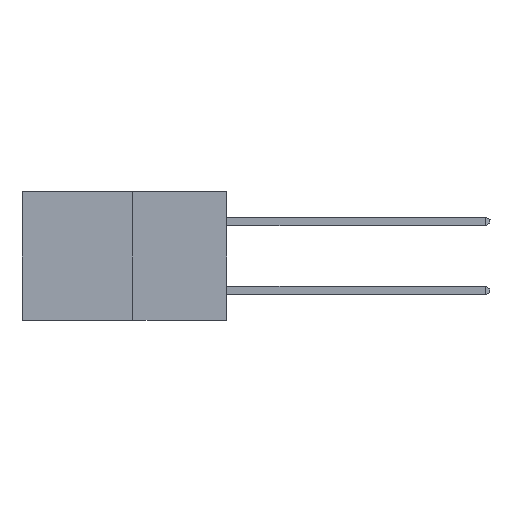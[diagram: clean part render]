
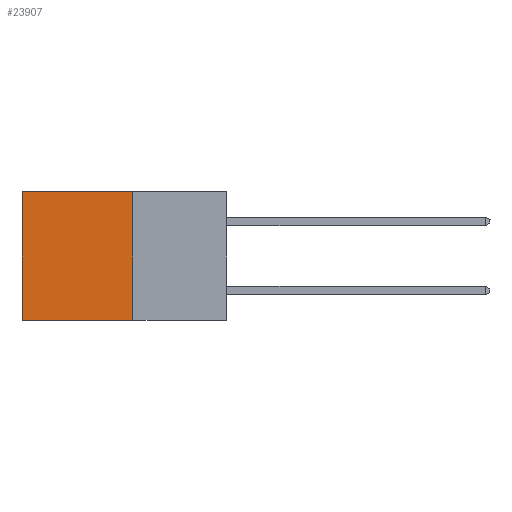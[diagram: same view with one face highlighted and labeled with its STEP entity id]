
A CAD part, left-side view. The second image highlights one B-rep face of the part: STEP entity #23907.
In plain terms, the highlighted planar face has unit normal (-1, 0, 0).
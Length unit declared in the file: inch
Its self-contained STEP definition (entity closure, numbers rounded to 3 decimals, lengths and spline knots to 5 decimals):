
#242 = DIRECTION ( 'NONE',  ( 0., 1., 0. ) ) ;
#1425 = EDGE_CURVE ( 'NONE', #26429, #18864, #28912, .T. ) ;
#3086 = VECTOR ( 'NONE', #17994, 39.37008 ) ;
#3312 = DIRECTION ( 'NONE',  ( 0., 1., 0. ) ) ;
#3523 = CARTESIAN_POINT ( 'NONE',  ( 0.277, 0.27, -0.37 ) ) ;
#3589 = VECTOR ( 'NONE', #14369, 39.37008 ) ;
#4187 = DIRECTION ( 'NONE',  ( 1., 0., 0. ) ) ;
#5069 = EDGE_CURVE ( 'NONE', #18864, #12966, #28674, .T. ) ;
#7683 = CARTESIAN_POINT ( 'NONE',  ( 0.277, 0.27, -0.37 ) ) ;
#8661 = CARTESIAN_POINT ( 'NONE',  ( 0.277, 0.59, -0.37 ) ) ;
#8936 = CARTESIAN_POINT ( 'NONE',  ( 0.277, 0.27, -0.37 ) ) ;
#10080 = VECTOR ( 'NONE', #3312, 39.37008 ) ;
#11378 = ORIENTED_EDGE ( 'NONE', *, *, #19986, .T. ) ;
#12966 = VERTEX_POINT ( 'NONE', #8661 ) ;
#13251 = AXIS2_PLACEMENT_3D ( 'NONE', #8936, #4187, #21246 ) ;
#14275 = CARTESIAN_POINT ( 'NONE',  ( 0.277, 0.27, 0. ) ) ;
#14369 = DIRECTION ( 'NONE',  ( 0., 0., -1. ) ) ;
#14559 = ORIENTED_EDGE ( 'NONE', *, *, #1425, .F. ) ;
#14977 = ORIENTED_EDGE ( 'NONE', *, *, #23497, .T. ) ;
#14979 = CARTESIAN_POINT ( 'NONE',  ( 0.277, 0.27, 0. ) ) ;
#17994 = DIRECTION ( 'NONE',  ( 0., 0., -1. ) ) ;
#18455 = CARTESIAN_POINT ( 'NONE',  ( 0.277, 0.27, -0.37 ) ) ;
#18764 = PLANE ( 'NONE',  #13251 ) ;
#18864 = VERTEX_POINT ( 'NONE', #7683 ) ;
#19803 = CARTESIAN_POINT ( 'NONE',  ( 0.277, 0.59, 0. ) ) ;
#19986 = EDGE_CURVE ( 'NONE', #26615, #12966, #28657, .T. ) ;
#20922 = LINE ( 'NONE', #14979, #22446 ) ;
#21246 = DIRECTION ( 'NONE',  ( 0., 0., -1. ) ) ;
#21377 = ORIENTED_EDGE ( 'NONE', *, *, #5069, .F. ) ;
#21657 = FACE_OUTER_BOUND ( 'NONE', #22285, .T. ) ;
#22285 = EDGE_LOOP ( 'NONE', ( #11378, #21377, #14559, #14977 ) ) ;
#22446 = VECTOR ( 'NONE', #242, 39.37008 ) ;
#23497 = EDGE_CURVE ( 'NONE', #26429, #26615, #20922, .T. ) ;
#23907 = ADVANCED_FACE ( 'NONE', ( #21657 ), #18764, .F. ) ;
#26429 = VERTEX_POINT ( 'NONE', #14275 ) ;
#26615 = VERTEX_POINT ( 'NONE', #19803 ) ;
#28657 = LINE ( 'NONE', #28850, #3589 ) ;
#28674 = LINE ( 'NONE', #3523, #10080 ) ;
#28850 = CARTESIAN_POINT ( 'NONE',  ( 0.277, 0.59, -0.37 ) ) ;
#28912 = LINE ( 'NONE', #18455, #3086 ) ;
